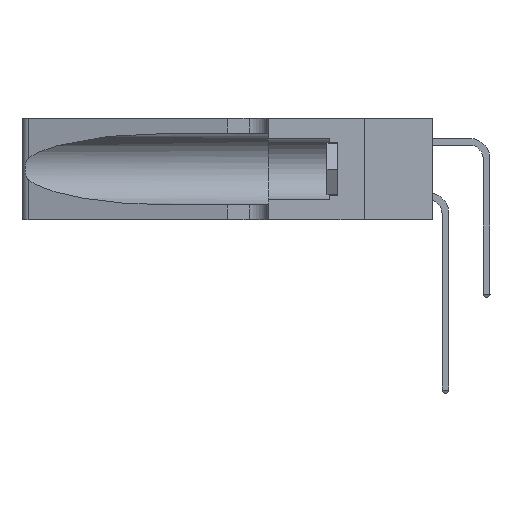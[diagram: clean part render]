
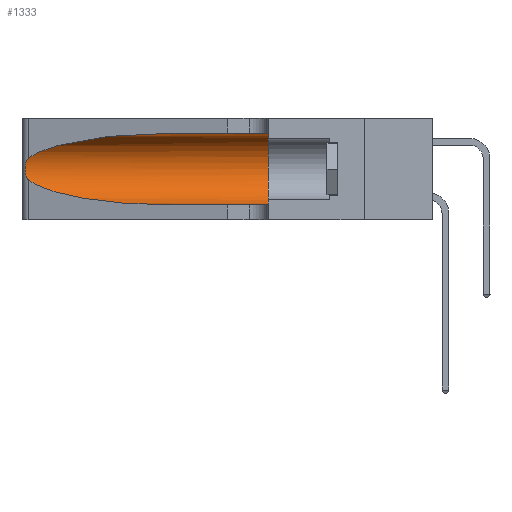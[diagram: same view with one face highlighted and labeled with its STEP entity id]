
A CAD part, left-side view. The second image highlights one B-rep face of the part: STEP entity #1333.
In plain terms, the highlighted cylindrical face has radius 3.308 mm (diameter 6.617 mm), a partial arc.
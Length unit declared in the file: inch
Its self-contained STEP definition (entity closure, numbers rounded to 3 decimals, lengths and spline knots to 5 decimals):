
#41 = ORIENTED_EDGE ( 'NONE', *, *, #8276, .T. ) ;
#589 = CARTESIAN_POINT ( 'NONE',  ( 0.1305, 0.72297, 0.05475 ) ) ;
#890 = ORIENTED_EDGE ( 'NONE', *, *, #17754, .T. ) ;
#1333 = ADVANCED_FACE ( 'NONE', ( #12133 ), #19305, .F. ) ;
#1812 = EDGE_CURVE ( 'NONE', #13376, #9978, #13755, .T. ) ;
#2103 = CARTESIAN_POINT ( 'NONE',  ( 0.25487, 1.22718, 0.14631 ) ) ;
#2171 = CARTESIAN_POINT ( 'NONE',  ( 0.26075, 1.23896, 0.19203 ) ) ;
#2247 = CARTESIAN_POINT ( 'NONE',  ( 0.25639, 1.23184, 0.21858 ) ) ;
#3630 = VECTOR ( 'NONE', #7529, 39.37008 ) ;
#3912 =( BOUNDED_CURVE ( )  B_SPLINE_CURVE ( 3, ( #17697, #12662, #17627, #8024 ),
 .UNSPECIFIED., .F., .F. ) 
 B_SPLINE_CURVE_WITH_KNOTS ( ( 4, 4 ),
 ( 3.44316, 4.71239 ),
 .UNSPECIFIED. ) 
 CURVE ( )  GEOMETRIC_REPRESENTATION_ITEM ( )  RATIONAL_B_SPLINE_CURVE ( ( 1., 0.87, 0.87, 1. ) ) 
 REPRESENTATION_ITEM ( '' )  );
#4305 = CARTESIAN_POINT ( 'NONE',  ( 0.18966, 0.96281, 0.31525 ) ) ;
#4392 = CARTESIAN_POINT ( 'NONE',  ( 0.1305, 0.72297, 0.31525 ) ) ;
#4703 = CARTESIAN_POINT ( 'NONE',  ( 0.25487, 1.22718, 0.22369 ) ) ;
#4804 = CARTESIAN_POINT ( 'NONE',  ( 0.25487, 1.22718, 0.14631 ) ) ;
#5333 = CARTESIAN_POINT ( 'NONE',  ( 0.25787, 1.23484, 0.2124 ) ) ;
#5520 = VERTEX_POINT ( 'NONE', #10190 ) ;
#5593 = LINE ( 'NONE', #12888, #18912 ) ;
#5618 = CARTESIAN_POINT ( 'NONE',  ( 0.25856, 1.23593, 0.16098 ) ) ;
#6045 = AXIS2_PLACEMENT_3D ( 'NONE', #10744, #18936, #12085 ) ;
#6105 = CARTESIAN_POINT ( 'NONE',  ( 0.25487, 1.22718, 0.22369 ) ) ;
#6324 = EDGE_CURVE ( 'NONE', #12571, #5520, #19541, .T. ) ;
#6340 = EDGE_CURVE ( 'NONE', #13376, #12571, #19286, .T. ) ;
#7113 = CARTESIAN_POINT ( 'NONE',  ( 0.25789, 1.23486, 0.15765 ) ) ;
#7184 = CARTESIAN_POINT ( 'NONE',  ( 0.25854, 1.2359, 0.20912 ) ) ;
#7250 = CARTESIAN_POINT ( 'NONE',  ( 0.25555, 1.22993, 0.14849 ) ) ;
#7480 = ORIENTED_EDGE ( 'NONE', *, *, #20069, .T. ) ;
#7529 = DIRECTION ( 'NONE',  ( 0., -1., 0. ) ) ;
#8024 = CARTESIAN_POINT ( 'NONE',  ( 0.1305, 0.72297, 0.05475 ) ) ;
#8276 = EDGE_CURVE ( 'NONE', #9439, #20157, #3912, .T. ) ;
#9170 = AXIS2_PLACEMENT_3D ( 'NONE', #18725, #15508, #13779 ) ;
#9439 = VERTEX_POINT ( 'NONE', #4804 ) ;
#9494 = CARTESIAN_POINT ( 'NONE',  ( 0.1305, 0.72297, 0.31525 ) ) ;
#9978 = VERTEX_POINT ( 'NONE', #4703 ) ;
#10190 = CARTESIAN_POINT ( 'NONE',  ( 0.1305, 0.35, 0.05475 ) ) ;
#10525 = CARTESIAN_POINT ( 'NONE',  ( 0.26017, 1.23833, 0.17102 ) ) ;
#10584 = CARTESIAN_POINT ( 'NONE',  ( 0.26018, 1.23835, 0.19895 ) ) ;
#10744 = CARTESIAN_POINT ( 'NONE',  ( 0.1305, 0.35, 0.185 ) ) ;
#11024 = CARTESIAN_POINT ( 'NONE',  ( 0.1305, 1.61858, 0.31525 ) ) ;
#11279 = ORIENTED_EDGE ( 'NONE', *, *, #6324, .F. ) ;
#11854 = ORIENTED_EDGE ( 'NONE', *, *, #1812, .T. ) ;
#11929 = CARTESIAN_POINT ( 'NONE',  ( 0.25487, 1.22718, 0.22369 ) ) ;
#12085 = DIRECTION ( 'NONE',  ( 0., 0., 1. ) ) ;
#12133 = FACE_OUTER_BOUND ( 'NONE', #17674, .T. ) ;
#12571 = VERTEX_POINT ( 'NONE', #14271 ) ;
#12662 = CARTESIAN_POINT ( 'NONE',  ( 0.2373, 1.15595, 0.08982 ) ) ;
#12888 = CARTESIAN_POINT ( 'NONE',  ( 0.1305, 1.61858, 0.05475 ) ) ;
#13376 = VERTEX_POINT ( 'NONE', #4392 ) ;
#13385 = DIRECTION ( 'NONE',  ( 0., -1., 0. ) ) ;
#13755 =( BOUNDED_CURVE ( )  B_SPLINE_CURVE ( 3, ( #9494, #4305, #15778, #6105 ),
 .UNSPECIFIED., .F., .T. ) 
 B_SPLINE_CURVE_WITH_KNOTS ( ( 4, 4 ),
 ( 1.5708, 2.84003 ),
 .UNSPECIFIED. ) 
 CURVE ( )  GEOMETRIC_REPRESENTATION_ITEM ( )  RATIONAL_B_SPLINE_CURVE ( ( 1., 0.87, 0.87, 1. ) ) 
 REPRESENTATION_ITEM ( '' )  );
#13779 = DIRECTION ( 'NONE',  ( 0., 0., -1. ) ) ;
#14271 = CARTESIAN_POINT ( 'NONE',  ( 0.1305, 0.35, 0.31525 ) ) ;
#14832 = ORIENTED_EDGE ( 'NONE', *, *, #6340, .F. ) ;
#15196 = CARTESIAN_POINT ( 'NONE',  ( 0.26075, 1.23896, 0.178 ) ) ;
#15508 = DIRECTION ( 'NONE',  ( 0., -1., 0. ) ) ;
#15778 = CARTESIAN_POINT ( 'NONE',  ( 0.2373, 1.15595, 0.28018 ) ) ;
#16876 = CARTESIAN_POINT ( 'NONE',  ( 0.25555, 1.22994, 0.2215 ) ) ;
#17081 = CARTESIAN_POINT ( 'NONE',  ( 0.25639, 1.23186, 0.15144 ) ) ;
#17627 = CARTESIAN_POINT ( 'NONE',  ( 0.18966, 0.96281, 0.05475 ) ) ;
#17674 = EDGE_LOOP ( 'NONE', ( #11854, #890, #41, #7480, #11279, #14832 ) ) ;
#17697 = CARTESIAN_POINT ( 'NONE',  ( 0.25487, 1.22718, 0.14631 ) ) ;
#17754 = EDGE_CURVE ( 'NONE', #9978, #9439, #18894, .T. ) ;
#18725 = CARTESIAN_POINT ( 'NONE',  ( 0.1305, 1.61858, 0.185 ) ) ;
#18894 = B_SPLINE_CURVE_WITH_KNOTS ( 'NONE', 3,
 ( #11929, #16876, #2247, #5333, #7184, #10584, #2171, #15196, #10525, #5618, #7113, #17081, #7250, #2103 ),
 .UNSPECIFIED., .F., .F.,
 ( 4, 2, 2, 2, 2, 2, 4 ),
 ( 0., 0.00027, 0.00053, 0.00107, 0.0016, 0.00187, 0.00214 ),
 .UNSPECIFIED. ) ;
#18912 = VECTOR ( 'NONE', #13385, 39.37008 ) ;
#18936 = DIRECTION ( 'NONE',  ( 0., 1., 0. ) ) ;
#19286 = LINE ( 'NONE', #11024, #3630 ) ;
#19305 = CYLINDRICAL_SURFACE ( 'NONE', #9170, 0.13025 ) ;
#19541 = CIRCLE ( 'NONE', #6045, 0.13025 ) ;
#20069 = EDGE_CURVE ( 'NONE', #20157, #5520, #5593, .T. ) ;
#20157 = VERTEX_POINT ( 'NONE', #589 ) ;
